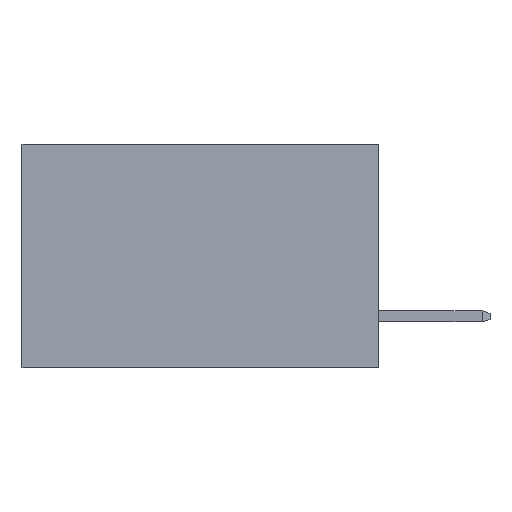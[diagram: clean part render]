
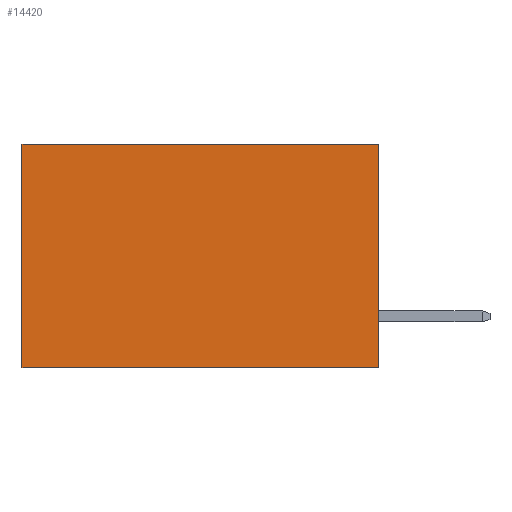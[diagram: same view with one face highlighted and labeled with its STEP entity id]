
A CAD part, left-side view. The second image highlights one B-rep face of the part: STEP entity #14420.
In plain terms, the highlighted planar face has unit normal (-1, 0, 0).
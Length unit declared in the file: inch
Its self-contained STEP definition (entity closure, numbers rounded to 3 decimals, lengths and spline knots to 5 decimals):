
#105 = VECTOR ( 'NONE', #14130, 39.37008 ) ;
#609 = EDGE_CURVE ( 'NONE', #2068, #2855, #11050, .T. ) ;
#2068 = VERTEX_POINT ( 'NONE', #7410 ) ;
#2157 = CARTESIAN_POINT ( 'NONE',  ( 0.277, 0.59, -0.37 ) ) ;
#2855 = VERTEX_POINT ( 'NONE', #19158 ) ;
#3620 = ORIENTED_EDGE ( 'NONE', *, *, #20214, .F. ) ;
#4050 = EDGE_CURVE ( 'NONE', #14314, #2855, #13214, .T. ) ;
#5089 = VERTEX_POINT ( 'NONE', #7299 ) ;
#5594 = DIRECTION ( 'NONE',  ( 1., 0., 0. ) ) ;
#6098 = ORIENTED_EDGE ( 'NONE', *, *, #4050, .F. ) ;
#6523 = CARTESIAN_POINT ( 'NONE',  ( 0.277, 0., -0.37 ) ) ;
#6651 = VECTOR ( 'NONE', #8213, 39.37008 ) ;
#6687 = VECTOR ( 'NONE', #12738, 39.37008 ) ;
#7299 = CARTESIAN_POINT ( 'NONE',  ( 0.277, 0., 0. ) ) ;
#7410 = CARTESIAN_POINT ( 'NONE',  ( 0.277, 0.59, 0. ) ) ;
#8213 = DIRECTION ( 'NONE',  ( 0., 0., -1. ) ) ;
#8562 = LINE ( 'NONE', #16525, #20836 ) ;
#9818 = AXIS2_PLACEMENT_3D ( 'NONE', #12116, #5594, #16925 ) ;
#9989 = CARTESIAN_POINT ( 'NONE',  ( 0.277, 0., -0.37 ) ) ;
#10137 = DIRECTION ( 'NONE',  ( 0., 1., 0. ) ) ;
#10573 = EDGE_LOOP ( 'NONE', ( #17446, #6098, #3620, #14571 ) ) ;
#11050 = LINE ( 'NONE', #2157, #6687 ) ;
#11153 = FACE_OUTER_BOUND ( 'NONE', #10573, .T. ) ;
#12116 = CARTESIAN_POINT ( 'NONE',  ( 0.277, 0., -0.37 ) ) ;
#12738 = DIRECTION ( 'NONE',  ( 0., 0., -1. ) ) ;
#13214 = LINE ( 'NONE', #9989, #105 ) ;
#13454 = CARTESIAN_POINT ( 'NONE',  ( 0.277, 0., -0.37 ) ) ;
#14130 = DIRECTION ( 'NONE',  ( 0., 1., 0. ) ) ;
#14314 = VERTEX_POINT ( 'NONE', #13454 ) ;
#14420 = ADVANCED_FACE ( 'NONE', ( #11153 ), #16858, .F. ) ;
#14571 = ORIENTED_EDGE ( 'NONE', *, *, #17635, .T. ) ;
#16525 = CARTESIAN_POINT ( 'NONE',  ( 0.277, 0., 0. ) ) ;
#16858 = PLANE ( 'NONE',  #9818 ) ;
#16925 = DIRECTION ( 'NONE',  ( 0., 0., -1. ) ) ;
#17446 = ORIENTED_EDGE ( 'NONE', *, *, #609, .T. ) ;
#17635 = EDGE_CURVE ( 'NONE', #5089, #2068, #8562, .T. ) ;
#19158 = CARTESIAN_POINT ( 'NONE',  ( 0.277, 0.59, -0.37 ) ) ;
#19994 = LINE ( 'NONE', #6523, #6651 ) ;
#20214 = EDGE_CURVE ( 'NONE', #5089, #14314, #19994, .T. ) ;
#20836 = VECTOR ( 'NONE', #10137, 39.37008 ) ;
